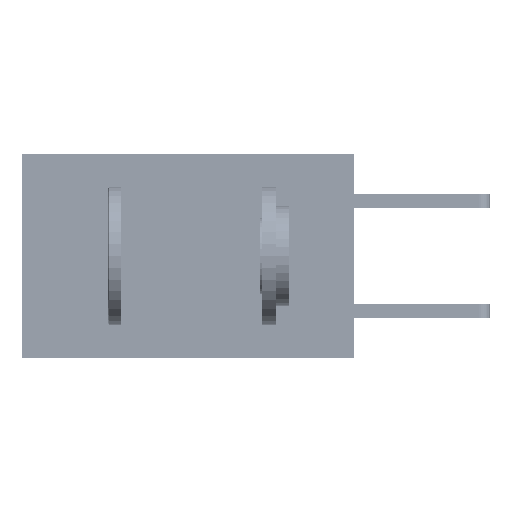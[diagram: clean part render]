
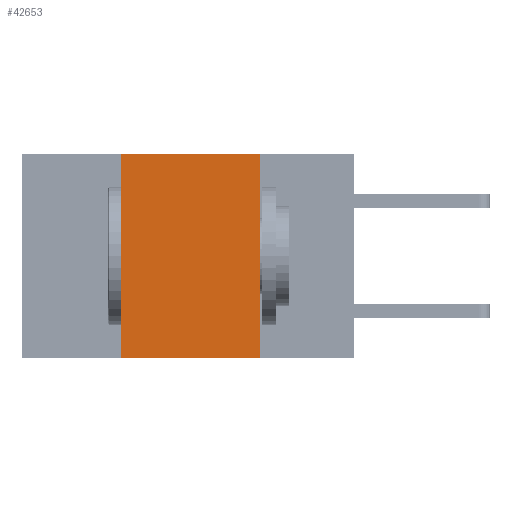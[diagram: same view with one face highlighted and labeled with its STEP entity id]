
A CAD part, left-side view. The second image highlights one B-rep face of the part: STEP entity #42653.
In plain terms, the highlighted planar face has unit normal (-1, 0, 0).
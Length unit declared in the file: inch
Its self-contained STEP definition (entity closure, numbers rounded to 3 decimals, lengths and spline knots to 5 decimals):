
#55 = EDGE_CURVE ( 'NONE', #4033, #14480, #29300, .T. ) ;
#411 = VECTOR ( 'NONE', #51133, 39.37008 ) ;
#757 = EDGE_CURVE ( 'NONE', #41499, #30643, #16951, .T. ) ;
#1094 = AXIS2_PLACEMENT_3D ( 'NONE', #1216, #9293, #34071 ) ;
#1216 = CARTESIAN_POINT ( 'NONE',  ( 0., 0.6, 0. ) ) ;
#2594 = CARTESIAN_POINT ( 'NONE',  ( 0., 0.6, -0.37 ) ) ;
#4033 = VERTEX_POINT ( 'NONE', #5052 ) ;
#5052 = CARTESIAN_POINT ( 'NONE',  ( 0., 0.42, 0. ) ) ;
#6029 = DIRECTION ( 'NONE',  ( 0., -1., 0. ) ) ;
#6240 = CARTESIAN_POINT ( 'NONE',  ( 0., 0.17, 0. ) ) ;
#6375 = EDGE_LOOP ( 'NONE', ( #49878, #43941, #9831, #21750 ) ) ;
#6509 = LINE ( 'NONE', #47920, #30870 ) ;
#9293 = DIRECTION ( 'NONE',  ( 1., 0., 0. ) ) ;
#9498 = FACE_OUTER_BOUND ( 'NONE', #6375, .T. ) ;
#9831 = ORIENTED_EDGE ( 'NONE', *, *, #34658, .F. ) ;
#10518 = CARTESIAN_POINT ( 'NONE',  ( 0., 0.42, 0. ) ) ;
#10643 = CARTESIAN_POINT ( 'NONE',  ( 0., 0.42, -0.37 ) ) ;
#14480 = VERTEX_POINT ( 'NONE', #6240 ) ;
#14728 = EDGE_CURVE ( 'NONE', #14480, #30643, #6509, .T. ) ;
#16951 = LINE ( 'NONE', #2594, #39490 ) ;
#19720 = VECTOR ( 'NONE', #22932, 39.37008 ) ;
#21092 = CARTESIAN_POINT ( 'NONE',  ( 0., 0.17, -0.37 ) ) ;
#21750 = ORIENTED_EDGE ( 'NONE', *, *, #757, .T. ) ;
#22932 = DIRECTION ( 'NONE',  ( 0., 0., 1. ) ) ;
#27381 = DIRECTION ( 'NONE',  ( 0., 0., -1. ) ) ;
#29300 = LINE ( 'NONE', #38914, #411 ) ;
#30643 = VERTEX_POINT ( 'NONE', #21092 ) ;
#30870 = VECTOR ( 'NONE', #27381, 39.37008 ) ;
#33854 = LINE ( 'NONE', #10518, #19720 ) ;
#34071 = DIRECTION ( 'NONE',  ( 0., 0., -1. ) ) ;
#34658 = EDGE_CURVE ( 'NONE', #41499, #4033, #33854, .T. ) ;
#38914 = CARTESIAN_POINT ( 'NONE',  ( 0., 0.6, 0. ) ) ;
#39490 = VECTOR ( 'NONE', #6029, 39.37008 ) ;
#41499 = VERTEX_POINT ( 'NONE', #10643 ) ;
#42004 = PLANE ( 'NONE',  #1094 ) ;
#42653 = ADVANCED_FACE ( 'NONE', ( #9498 ), #42004, .F. ) ;
#43941 = ORIENTED_EDGE ( 'NONE', *, *, #55, .F. ) ;
#47920 = CARTESIAN_POINT ( 'NONE',  ( 0., 0.17, 0. ) ) ;
#49878 = ORIENTED_EDGE ( 'NONE', *, *, #14728, .F. ) ;
#51133 = DIRECTION ( 'NONE',  ( 0., -1., 0. ) ) ;
